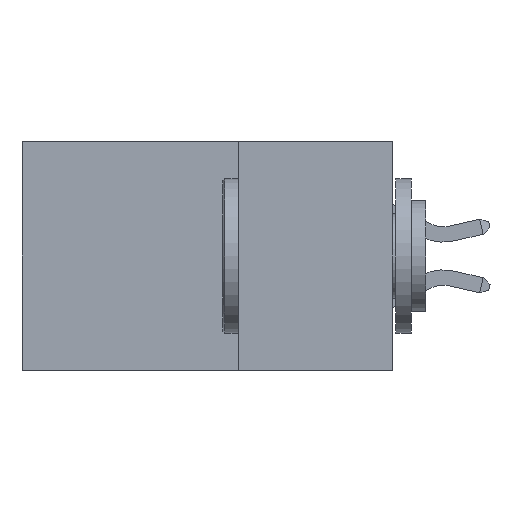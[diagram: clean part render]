
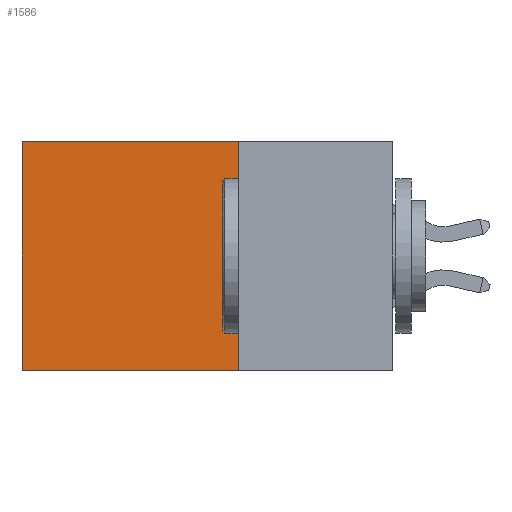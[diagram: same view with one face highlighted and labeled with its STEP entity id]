
A CAD part, left-side view. The second image highlights one B-rep face of the part: STEP entity #1586.
In plain terms, the highlighted planar face has unit normal (-1, 0, 0).
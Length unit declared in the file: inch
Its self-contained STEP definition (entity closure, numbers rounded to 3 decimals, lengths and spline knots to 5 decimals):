
#184 = VERTEX_POINT ( 'NONE', #3821 ) ;
#873 = EDGE_CURVE ( 'NONE', #184, #22744, #1521, .T. ) ;
#875 = ORIENTED_EDGE ( 'NONE', *, *, #873, .T. ) ;
#1521 = LINE ( 'NONE', #18780, #7259 ) ;
#1586 = ADVANCED_FACE ( 'NONE', ( #19976 ), #22085, .F. ) ;
#1737 = AXIS2_PLACEMENT_3D ( 'NONE', #22192, #16795, #24985 ) ;
#2643 = EDGE_CURVE ( 'NONE', #12599, #184, #18709, .T. ) ;
#3821 = CARTESIAN_POINT ( 'NONE',  ( 0.2875, 0.6, 0. ) ) ;
#4769 = VERTEX_POINT ( 'NONE', #10523 ) ;
#5756 = CARTESIAN_POINT ( 'NONE',  ( 0.2875, 0.25, 0. ) ) ;
#7051 = EDGE_CURVE ( 'NONE', #4769, #22744, #29835, .T. ) ;
#7259 = VECTOR ( 'NONE', #26211, 39.37008 ) ;
#10188 = CARTESIAN_POINT ( 'NONE',  ( 0.2875, 0.6, -0.37 ) ) ;
#10254 = DIRECTION ( 'NONE',  ( 0., 1., 0. ) ) ;
#10523 = CARTESIAN_POINT ( 'NONE',  ( 0.2875, 0.25, -0.37 ) ) ;
#12219 = ORIENTED_EDGE ( 'NONE', *, *, #15055, .F. ) ;
#12599 = VERTEX_POINT ( 'NONE', #5756 ) ;
#12819 = CARTESIAN_POINT ( 'NONE',  ( 0.2875, 0.25, -0.37 ) ) ;
#13726 = LINE ( 'NONE', #21335, #21070 ) ;
#15055 = EDGE_CURVE ( 'NONE', #12599, #4769, #13726, .T. ) ;
#15339 = CARTESIAN_POINT ( 'NONE',  ( 0.2875, 0.25, 0. ) ) ;
#15627 = VECTOR ( 'NONE', #10254, 39.37008 ) ;
#16795 = DIRECTION ( 'NONE',  ( 1., 0., 0. ) ) ;
#17481 = VECTOR ( 'NONE', #30048, 39.37008 ) ;
#18355 = ORIENTED_EDGE ( 'NONE', *, *, #2643, .T. ) ;
#18465 = ORIENTED_EDGE ( 'NONE', *, *, #7051, .F. ) ;
#18709 = LINE ( 'NONE', #15339, #15627 ) ;
#18780 = CARTESIAN_POINT ( 'NONE',  ( 0.2875, 0.6, 0. ) ) ;
#19976 = FACE_OUTER_BOUND ( 'NONE', #28707, .T. ) ;
#21070 = VECTOR ( 'NONE', #31349, 39.37008 ) ;
#21335 = CARTESIAN_POINT ( 'NONE',  ( 0.2875, 0.25, 0. ) ) ;
#22085 = PLANE ( 'NONE',  #1737 ) ;
#22192 = CARTESIAN_POINT ( 'NONE',  ( 0.2875, 0.25, 0. ) ) ;
#22744 = VERTEX_POINT ( 'NONE', #10188 ) ;
#24985 = DIRECTION ( 'NONE',  ( 0., 0., -1. ) ) ;
#26211 = DIRECTION ( 'NONE',  ( 0., 0., -1. ) ) ;
#28707 = EDGE_LOOP ( 'NONE', ( #875, #18465, #12219, #18355 ) ) ;
#29835 = LINE ( 'NONE', #12819, #17481 ) ;
#30048 = DIRECTION ( 'NONE',  ( 0., 1., 0. ) ) ;
#31349 = DIRECTION ( 'NONE',  ( 0., 0., -1. ) ) ;
